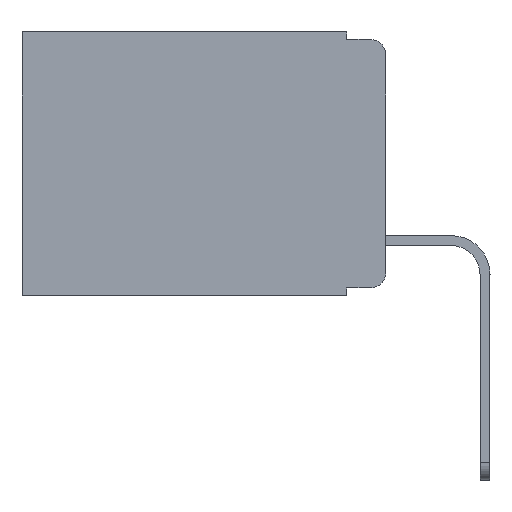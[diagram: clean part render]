
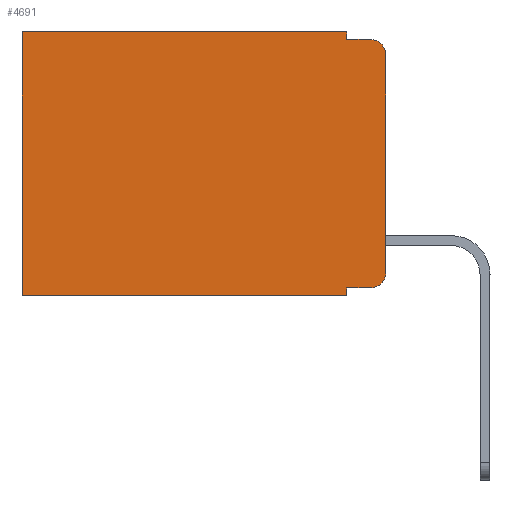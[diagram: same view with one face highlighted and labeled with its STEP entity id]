
A CAD part, left-side view. The second image highlights one B-rep face of the part: STEP entity #4691.
In plain terms, the highlighted planar face has unit normal (-1, 0, 0).
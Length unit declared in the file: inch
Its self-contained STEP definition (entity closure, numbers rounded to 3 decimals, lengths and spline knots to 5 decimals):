
#6 = LINE ( 'NONE', #6828, #9088 ) ;
#210 = LINE ( 'NONE', #6215, #7867 ) ;
#444 = AXIS2_PLACEMENT_3D ( 'NONE', #2928, #13443, #10447 ) ;
#738 = EDGE_CURVE ( 'NONE', #16111, #5163, #19353, .T. ) ;
#1453 = VERTEX_POINT ( 'NONE', #13596 ) ;
#1629 = VECTOR ( 'NONE', #14457, 39.37008 ) ;
#1704 = DIRECTION ( 'NONE',  ( 0., 0., -1. ) ) ;
#1719 = CARTESIAN_POINT ( 'NONE',  ( 0.298, 0.051, -0.01 ) ) ;
#1762 = DIRECTION ( 'NONE',  ( -1., 0., 0. ) ) ;
#2242 = CARTESIAN_POINT ( 'NONE',  ( 0.298, 0.051, -0.333 ) ) ;
#2461 = EDGE_CURVE ( 'NONE', #16111, #14028, #6, .T. ) ;
#2582 = DIRECTION ( 'NONE',  ( 0., 1., 0. ) ) ;
#2611 = CARTESIAN_POINT ( 'NONE',  ( 0.298, 0., -0.313 ) ) ;
#2630 = VECTOR ( 'NONE', #10979, 39.37008 ) ;
#2928 = CARTESIAN_POINT ( 'NONE',  ( 0.298, 0., 0. ) ) ;
#3096 = VECTOR ( 'NONE', #11288, 39.37008 ) ;
#3233 = CARTESIAN_POINT ( 'NONE',  ( 0.298, 0.02, -0.03 ) ) ;
#3612 = AXIS2_PLACEMENT_3D ( 'NONE', #3233, #1762, #1704 ) ;
#4274 = VECTOR ( 'NONE', #15570, 39.37008 ) ;
#4547 = DIRECTION ( 'NONE',  ( 0., 0., -1. ) ) ;
#4587 = VERTEX_POINT ( 'NONE', #15863 ) ;
#4691 = ADVANCED_FACE ( 'NONE', ( #8040 ), #5816, .F. ) ;
#4948 = CIRCLE ( 'NONE', #5155, 0.02 ) ;
#5155 = AXIS2_PLACEMENT_3D ( 'NONE', #14509, #10080, #8366 ) ;
#5163 = VERTEX_POINT ( 'NONE', #17490 ) ;
#5214 = ORIENTED_EDGE ( 'NONE', *, *, #738, .T. ) ;
#5306 = ORIENTED_EDGE ( 'NONE', *, *, #17146, .T. ) ;
#5491 = ORIENTED_EDGE ( 'NONE', *, *, #15245, .T. ) ;
#5816 = PLANE ( 'NONE',  #444 ) ;
#6027 = DIRECTION ( 'NONE',  ( 0., 1., 0. ) ) ;
#6028 = CARTESIAN_POINT ( 'NONE',  ( 0.298, 0.051, 0. ) ) ;
#6215 = CARTESIAN_POINT ( 'NONE',  ( 0.298, 0., 0. ) ) ;
#6264 = CARTESIAN_POINT ( 'NONE',  ( 0.298, 0.02, -0.333 ) ) ;
#6708 = LINE ( 'NONE', #8210, #3096 ) ;
#6828 = CARTESIAN_POINT ( 'NONE',  ( 0.298, 0.051, 0. ) ) ;
#7504 = EDGE_CURVE ( 'NONE', #4587, #14946, #210, .T. ) ;
#7867 = VECTOR ( 'NONE', #4547, 39.37008 ) ;
#8040 = FACE_OUTER_BOUND ( 'NONE', #10521, .T. ) ;
#8210 = CARTESIAN_POINT ( 'NONE',  ( 0.298, 0.473, 0. ) ) ;
#8357 = LINE ( 'NONE', #15530, #2630 ) ;
#8366 = DIRECTION ( 'NONE',  ( 0., 0., -1. ) ) ;
#8659 = CARTESIAN_POINT ( 'NONE',  ( 0.298, 0., 0. ) ) ;
#8768 = EDGE_CURVE ( 'NONE', #12817, #9491, #8357, .T. ) ;
#8883 = ORIENTED_EDGE ( 'NONE', *, *, #12583, .T. ) ;
#9088 = VECTOR ( 'NONE', #9926, 39.37008 ) ;
#9260 = CARTESIAN_POINT ( 'NONE',  ( 0.298, 0.02, -0.01 ) ) ;
#9491 = VERTEX_POINT ( 'NONE', #17520 ) ;
#9750 = LINE ( 'NONE', #2242, #1629 ) ;
#9926 = DIRECTION ( 'NONE',  ( 0., 0., -1. ) ) ;
#10080 = DIRECTION ( 'NONE',  ( -1., 0., 0. ) ) ;
#10447 = DIRECTION ( 'NONE',  ( 0., 0., -1. ) ) ;
#10521 = EDGE_LOOP ( 'NONE', ( #13841, #16782, #17465, #16895, #5214, #5491, #16539, #13622, #5306, #8883 ) ) ;
#10979 = DIRECTION ( 'NONE',  ( 0., 0., -1. ) ) ;
#11288 = DIRECTION ( 'NONE',  ( 0., 0., -1. ) ) ;
#11848 = VERTEX_POINT ( 'NONE', #6264 ) ;
#11857 = EDGE_CURVE ( 'NONE', #14028, #15630, #18023, .T. ) ;
#12093 = CARTESIAN_POINT ( 'NONE',  ( 0.298, 0.051, -0.333 ) ) ;
#12304 = EDGE_CURVE ( 'NONE', #4587, #15630, #15834, .T. ) ;
#12583 = EDGE_CURVE ( 'NONE', #11848, #14946, #4948, .T. ) ;
#12817 = VERTEX_POINT ( 'NONE', #12093 ) ;
#12837 = EDGE_CURVE ( 'NONE', #9491, #1453, #15593, .T. ) ;
#13443 = DIRECTION ( 'NONE',  ( 1., 0., 0. ) ) ;
#13596 = CARTESIAN_POINT ( 'NONE',  ( 0.298, 0.473, -0.343 ) ) ;
#13622 = ORIENTED_EDGE ( 'NONE', *, *, #8768, .F. ) ;
#13841 = ORIENTED_EDGE ( 'NONE', *, *, #7504, .F. ) ;
#14028 = VERTEX_POINT ( 'NONE', #15442 ) ;
#14457 = DIRECTION ( 'NONE',  ( 0., -1., 0. ) ) ;
#14509 = CARTESIAN_POINT ( 'NONE',  ( 0.298, 0.02, -0.313 ) ) ;
#14653 = VECTOR ( 'NONE', #6027, 39.37008 ) ;
#14946 = VERTEX_POINT ( 'NONE', #2611 ) ;
#15245 = EDGE_CURVE ( 'NONE', #5163, #1453, #6708, .T. ) ;
#15308 = VECTOR ( 'NONE', #2582, 39.37008 ) ;
#15442 = CARTESIAN_POINT ( 'NONE',  ( 0.298, 0.051, -0.01 ) ) ;
#15530 = CARTESIAN_POINT ( 'NONE',  ( 0.298, 0.051, 0. ) ) ;
#15570 = DIRECTION ( 'NONE',  ( 0., -1., 0. ) ) ;
#15593 = LINE ( 'NONE', #18350, #14653 ) ;
#15630 = VERTEX_POINT ( 'NONE', #9260 ) ;
#15834 = CIRCLE ( 'NONE', #3612, 0.02 ) ;
#15863 = CARTESIAN_POINT ( 'NONE',  ( 0.298, 0., -0.03 ) ) ;
#16111 = VERTEX_POINT ( 'NONE', #6028 ) ;
#16539 = ORIENTED_EDGE ( 'NONE', *, *, #12837, .F. ) ;
#16782 = ORIENTED_EDGE ( 'NONE', *, *, #12304, .T. ) ;
#16895 = ORIENTED_EDGE ( 'NONE', *, *, #2461, .F. ) ;
#17146 = EDGE_CURVE ( 'NONE', #12817, #11848, #9750, .T. ) ;
#17465 = ORIENTED_EDGE ( 'NONE', *, *, #11857, .F. ) ;
#17490 = CARTESIAN_POINT ( 'NONE',  ( 0.298, 0.473, 0. ) ) ;
#17520 = CARTESIAN_POINT ( 'NONE',  ( 0.298, 0.051, -0.343 ) ) ;
#18023 = LINE ( 'NONE', #1719, #4274 ) ;
#18350 = CARTESIAN_POINT ( 'NONE',  ( 0.298, 0., -0.343 ) ) ;
#19353 = LINE ( 'NONE', #8659, #15308 ) ;
